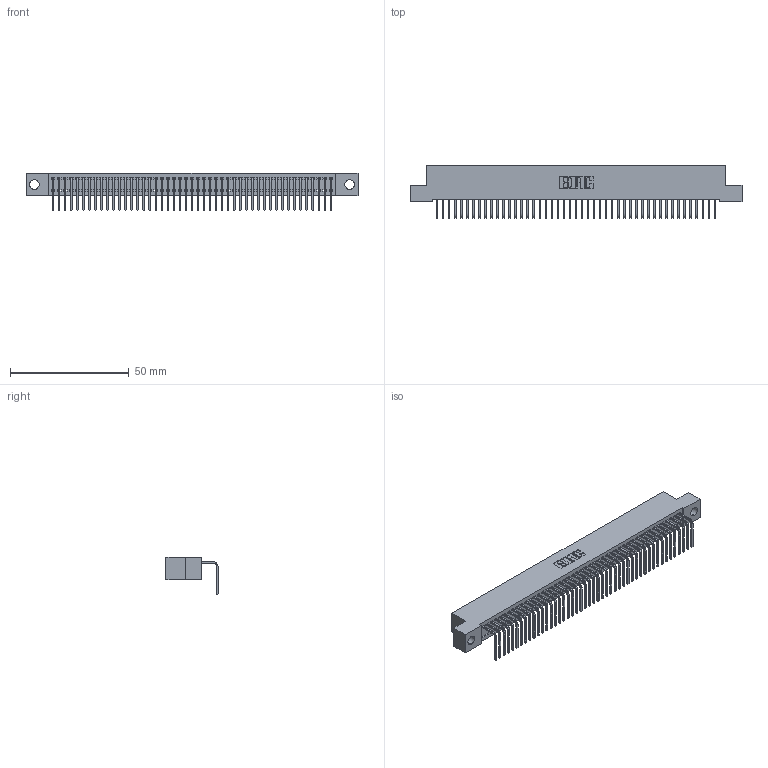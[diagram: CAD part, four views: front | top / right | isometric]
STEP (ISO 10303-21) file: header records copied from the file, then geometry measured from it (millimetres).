
FILE_DESCRIPTION (( 'STEP AP203' ), '1' );
FILE_NAME ('342-047-558-104.STEP', '2018-08-12T17:17:42', ( '' ), ( '' ), 'SwSTEP 2.0', 'SolidWorks 2016', '' );
FILE_SCHEMA (( 'CONFIG_CONTROL_DESIGN' ));
Length unit declared in the file: inch
Products named in the file (3): 345-292-001_558 Tail - 2; 342-047-558-104; 342 Part_.156 TH
Assembly tree (48 placements, depth 2):
  342-047-558-104
    342 Part_.156 TH
    345-292-001_558 Tail - 2  x47
Bounding box: 139.7 x 21.91 x 15.62 mm (x, y, z)
Volume: 12336.9 mm3; surface area: 18917.6 mm2
Topology: 48 solids, 48 shells, 2930 faces, 8853 edges, 5838 vertices
Faces by surface type: plane 2134, cylinder 796
Entity records: 28041 total; most frequent: CARTESIAN_POINT 4843, ORIENTED_EDGE 4826, DIRECTION 4075, EDGE_CURVE 2413, LINE 2285, VECTOR 2285, VERTEX_POINT 1606, AXIS2_PLACEMENT_3D 895
